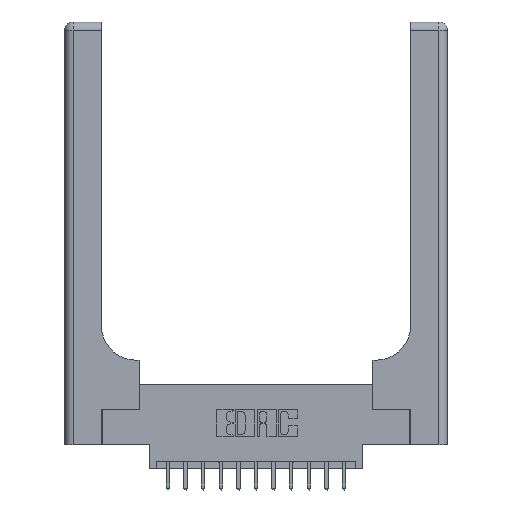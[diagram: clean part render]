
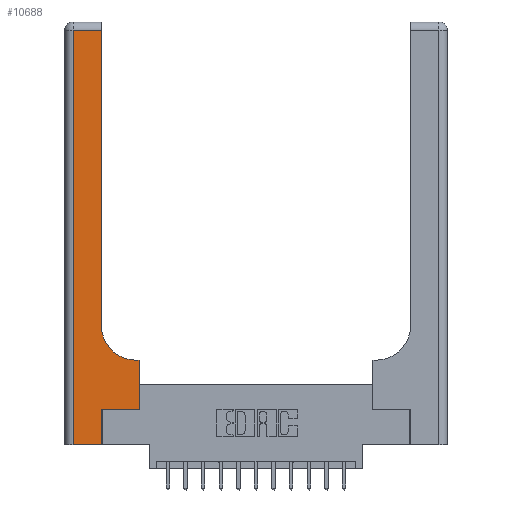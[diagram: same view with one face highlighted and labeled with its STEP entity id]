
A CAD part, top view. The second image highlights one B-rep face of the part: STEP entity #10688.
In plain terms, the highlighted planar face has unit normal (0, 0, 1).
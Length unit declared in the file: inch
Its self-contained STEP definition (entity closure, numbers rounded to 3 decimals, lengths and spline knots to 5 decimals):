
#179 = LINE ( 'NONE', #2970, #9054 ) ;
#256 = CARTESIAN_POINT ( 'NONE',  ( 0.265, 0., 0.37 ) ) ;
#267 = VECTOR ( 'NONE', #2784, 39.37008 ) ;
#348 = CARTESIAN_POINT ( 'NONE',  ( 0.265, 0.25, 0.37 ) ) ;
#717 = VECTOR ( 'NONE', #10278, 39.37008 ) ;
#1551 = CARTESIAN_POINT ( 'NONE',  ( 0.06, 2.94, 0.37 ) ) ;
#1746 = VERTEX_POINT ( 'NONE', #7737 ) ;
#1855 = VECTOR ( 'NONE', #11004, 39.37008 ) ;
#1890 = VERTEX_POINT ( 'NONE', #6713 ) ;
#1920 = EDGE_CURVE ( 'NONE', #5752, #7502, #179, .T. ) ;
#2380 = CARTESIAN_POINT ( 'NONE',  ( 0.528, 0.25, 0.37 ) ) ;
#2784 = DIRECTION ( 'NONE',  ( -1., 0., 0. ) ) ;
#2791 = EDGE_CURVE ( 'NONE', #15557, #15123, #8384, .T. ) ;
#2970 = CARTESIAN_POINT ( 'NONE',  ( 0.26, 0.6, 0.37 ) ) ;
#4050 = CARTESIAN_POINT ( 'NONE',  ( 0.51, 0.6, 0.37 ) ) ;
#4240 = DIRECTION ( 'NONE',  ( 0., 0., -1. ) ) ;
#4331 = DIRECTION ( 'NONE',  ( 1., 0., 0. ) ) ;
#4493 = CARTESIAN_POINT ( 'NONE',  ( 0., 3., 0.37 ) ) ;
#5208 = LINE ( 'NONE', #7621, #717 ) ;
#5714 = FACE_OUTER_BOUND ( 'NONE', #7619, .T. ) ;
#5752 = VERTEX_POINT ( 'NONE', #11183 ) ;
#5984 = ORIENTED_EDGE ( 'NONE', *, *, #2791, .T. ) ;
#6057 = ORIENTED_EDGE ( 'NONE', *, *, #15660, .T. ) ;
#6375 = AXIS2_PLACEMENT_3D ( 'NONE', #11766, #12687, #9898 ) ;
#6406 = VECTOR ( 'NONE', #10909, 39.37008 ) ;
#6713 = CARTESIAN_POINT ( 'NONE',  ( 0.265, 0., 0.37 ) ) ;
#6786 = CARTESIAN_POINT ( 'NONE',  ( 0., 2.94, 0.37 ) ) ;
#7059 = CARTESIAN_POINT ( 'NONE',  ( 0.528, 0.25, 0.37 ) ) ;
#7394 = VECTOR ( 'NONE', #14337, 39.37008 ) ;
#7502 = VERTEX_POINT ( 'NONE', #4050 ) ;
#7619 = EDGE_LOOP ( 'NONE', ( #15422, #14299, #8815, #12137, #6057, #5984, #16760, #15404, #7925 ) ) ;
#7621 = CARTESIAN_POINT ( 'NONE',  ( 0.26, 3., 0.37 ) ) ;
#7737 = CARTESIAN_POINT ( 'NONE',  ( 0.26, 0.85, 0.37 ) ) ;
#7925 = ORIENTED_EDGE ( 'NONE', *, *, #13806, .T. ) ;
#8013 = EDGE_CURVE ( 'NONE', #15123, #5752, #15098, .T. ) ;
#8382 = PLANE ( 'NONE',  #11488 ) ;
#8384 = LINE ( 'NONE', #16348, #11011 ) ;
#8714 = VERTEX_POINT ( 'NONE', #1551 ) ;
#8815 = ORIENTED_EDGE ( 'NONE', *, *, #13007, .T. ) ;
#8895 = CARTESIAN_POINT ( 'NONE',  ( 0., 0., 0.37 ) ) ;
#9054 = VECTOR ( 'NONE', #10580, 39.37008 ) ;
#9061 = LINE ( 'NONE', #8895, #7394 ) ;
#9876 = CARTESIAN_POINT ( 'NONE',  ( 0.06, 3., 0.37 ) ) ;
#9898 = DIRECTION ( 'NONE',  ( 1., 0., 0. ) ) ;
#10278 = DIRECTION ( 'NONE',  ( 0., 1., 0. ) ) ;
#10580 = DIRECTION ( 'NONE',  ( -1., 0., 0. ) ) ;
#10688 = ADVANCED_FACE ( 'NONE', ( #5714 ), #8382, .F. ) ;
#10909 = DIRECTION ( 'NONE',  ( 0., 1., 0. ) ) ;
#11004 = DIRECTION ( 'NONE',  ( 0., -1., 0. ) ) ;
#11011 = VECTOR ( 'NONE', #4331, 39.37008 ) ;
#11183 = CARTESIAN_POINT ( 'NONE',  ( 0.528, 0.6, 0.37 ) ) ;
#11424 = VECTOR ( 'NONE', #12326, 39.37008 ) ;
#11488 = AXIS2_PLACEMENT_3D ( 'NONE', #4493, #4240, #13591 ) ;
#11766 = CARTESIAN_POINT ( 'NONE',  ( 0.51, 0.85, 0.37 ) ) ;
#12046 = EDGE_CURVE ( 'NONE', #1746, #14425, #5208, .T. ) ;
#12137 = ORIENTED_EDGE ( 'NONE', *, *, #12521, .T. ) ;
#12326 = DIRECTION ( 'NONE',  ( 0., 1., 0. ) ) ;
#12521 = EDGE_CURVE ( 'NONE', #13474, #1890, #9061, .T. ) ;
#12665 = CARTESIAN_POINT ( 'NONE',  ( 0.26, 2.94, 0.37 ) ) ;
#12687 = DIRECTION ( 'NONE',  ( 0., 0., -1. ) ) ;
#13007 = EDGE_CURVE ( 'NONE', #8714, #13474, #16556, .T. ) ;
#13474 = VERTEX_POINT ( 'NONE', #13524 ) ;
#13524 = CARTESIAN_POINT ( 'NONE',  ( 0.06, 0., 0.37 ) ) ;
#13591 = DIRECTION ( 'NONE',  ( -1., 0., 0. ) ) ;
#13806 = EDGE_CURVE ( 'NONE', #7502, #1746, #16305, .T. ) ;
#14299 = ORIENTED_EDGE ( 'NONE', *, *, #14609, .T. ) ;
#14337 = DIRECTION ( 'NONE',  ( 1., 0., 0. ) ) ;
#14425 = VERTEX_POINT ( 'NONE', #12665 ) ;
#14609 = EDGE_CURVE ( 'NONE', #14425, #8714, #14638, .T. ) ;
#14638 = LINE ( 'NONE', #6786, #267 ) ;
#15098 = LINE ( 'NONE', #7059, #11424 ) ;
#15123 = VERTEX_POINT ( 'NONE', #2380 ) ;
#15160 = LINE ( 'NONE', #256, #6406 ) ;
#15404 = ORIENTED_EDGE ( 'NONE', *, *, #1920, .T. ) ;
#15422 = ORIENTED_EDGE ( 'NONE', *, *, #12046, .T. ) ;
#15557 = VERTEX_POINT ( 'NONE', #348 ) ;
#15660 = EDGE_CURVE ( 'NONE', #1890, #15557, #15160, .T. ) ;
#16305 = CIRCLE ( 'NONE', #6375, 0.25 ) ;
#16348 = CARTESIAN_POINT ( 'NONE',  ( 0.265, 0.25, 0.37 ) ) ;
#16556 = LINE ( 'NONE', #9876, #1855 ) ;
#16760 = ORIENTED_EDGE ( 'NONE', *, *, #8013, .T. ) ;
